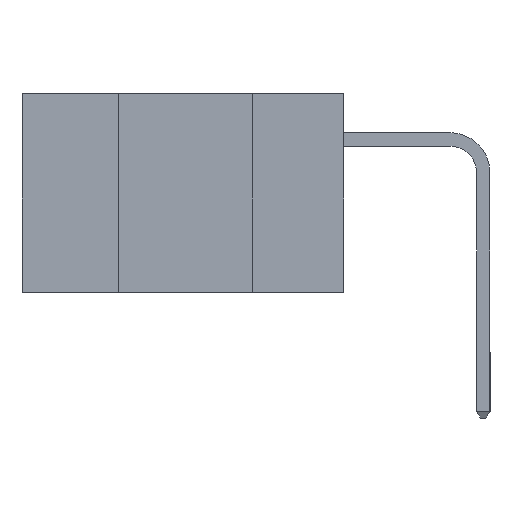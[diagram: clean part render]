
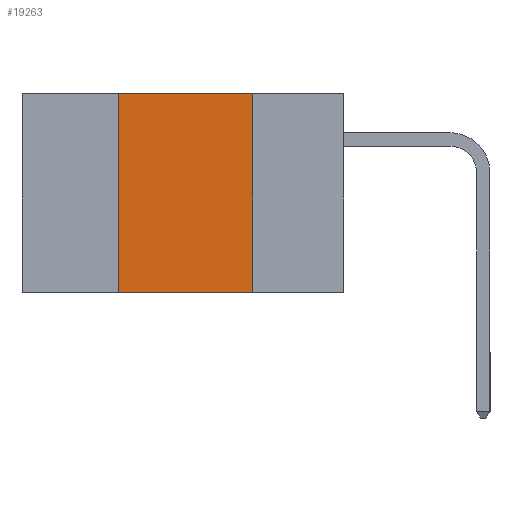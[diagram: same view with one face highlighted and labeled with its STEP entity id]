
A CAD part, left-side view. The second image highlights one B-rep face of the part: STEP entity #19263.
In plain terms, the highlighted planar face has unit normal (-1, 0, 0).
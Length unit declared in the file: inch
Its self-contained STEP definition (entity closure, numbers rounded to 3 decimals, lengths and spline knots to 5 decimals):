
#473 = VECTOR ( 'NONE', #15538, 39.37008 ) ;
#584 = VECTOR ( 'NONE', #9810, 39.37008 ) ;
#2471 = CARTESIAN_POINT ( 'NONE',  ( 0., 0.6, 0. ) ) ;
#3267 = CARTESIAN_POINT ( 'NONE',  ( 0., 0.42, 0. ) ) ;
#3332 = LINE ( 'NONE', #23368, #473 ) ;
#3589 = EDGE_CURVE ( 'NONE', #24962, #11645, #4324, .T. ) ;
#4324 = LINE ( 'NONE', #19343, #22907 ) ;
#5425 = PLANE ( 'NONE',  #11330 ) ;
#6776 = ORIENTED_EDGE ( 'NONE', *, *, #7344, .F. ) ;
#7344 = EDGE_CURVE ( 'NONE', #11573, #11645, #3332, .T. ) ;
#8418 = CARTESIAN_POINT ( 'NONE',  ( 0., 0.42, -0.37 ) ) ;
#9254 = EDGE_CURVE ( 'NONE', #24962, #18598, #14075, .T. ) ;
#9585 = DIRECTION ( 'NONE',  ( 0., -1., 0. ) ) ;
#9810 = DIRECTION ( 'NONE',  ( 0., -1., 0. ) ) ;
#10071 = LINE ( 'NONE', #2471, #584 ) ;
#10366 = VECTOR ( 'NONE', #18067, 39.37008 ) ;
#10555 = CARTESIAN_POINT ( 'NONE',  ( 0., 0.17, 0. ) ) ;
#11056 = CARTESIAN_POINT ( 'NONE',  ( 0., 0.17, -0.37 ) ) ;
#11330 = AXIS2_PLACEMENT_3D ( 'NONE', #23137, #13256, #21087 ) ;
#11573 = VERTEX_POINT ( 'NONE', #10555 ) ;
#11645 = VERTEX_POINT ( 'NONE', #11056 ) ;
#13256 = DIRECTION ( 'NONE',  ( 1., 0., 0. ) ) ;
#13973 = CARTESIAN_POINT ( 'NONE',  ( 0., 0.42, -0.37 ) ) ;
#14001 = ORIENTED_EDGE ( 'NONE', *, *, #3589, .T. ) ;
#14075 = LINE ( 'NONE', #8418, #10366 ) ;
#15538 = DIRECTION ( 'NONE',  ( 0., 0., -1. ) ) ;
#16754 = EDGE_CURVE ( 'NONE', #18598, #11573, #10071, .T. ) ;
#18067 = DIRECTION ( 'NONE',  ( 0., 0., 1. ) ) ;
#18598 = VERTEX_POINT ( 'NONE', #3267 ) ;
#19263 = ADVANCED_FACE ( 'NONE', ( #23020 ), #5425, .F. ) ;
#19343 = CARTESIAN_POINT ( 'NONE',  ( 0., 0.6, -0.37 ) ) ;
#20788 = EDGE_LOOP ( 'NONE', ( #6776, #23035, #23088, #14001 ) ) ;
#21087 = DIRECTION ( 'NONE',  ( 0., 0., -1. ) ) ;
#22907 = VECTOR ( 'NONE', #9585, 39.37008 ) ;
#23020 = FACE_OUTER_BOUND ( 'NONE', #20788, .T. ) ;
#23035 = ORIENTED_EDGE ( 'NONE', *, *, #16754, .F. ) ;
#23088 = ORIENTED_EDGE ( 'NONE', *, *, #9254, .F. ) ;
#23137 = CARTESIAN_POINT ( 'NONE',  ( 0., 0.6, 0. ) ) ;
#23368 = CARTESIAN_POINT ( 'NONE',  ( 0., 0.17, -0.37 ) ) ;
#24962 = VERTEX_POINT ( 'NONE', #13973 ) ;
